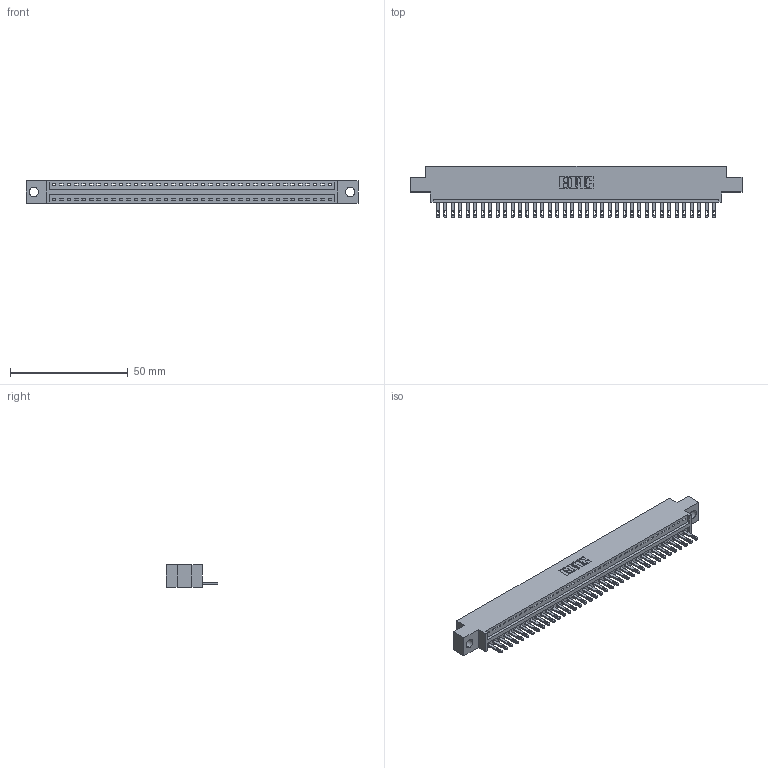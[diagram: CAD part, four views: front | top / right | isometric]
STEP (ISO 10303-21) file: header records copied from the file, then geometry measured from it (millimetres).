
FILE_DESCRIPTION (( 'STEP AP203' ), '1' );
FILE_NAME ('346-038-500-604.STEP', '2022-05-07T04:03:20', ( '' ), ( '' ), 'SwSTEP 2.0', 'SolidWorks 2020', '' );
FILE_SCHEMA (( 'CONFIG_CONTROL_DESIGN' ));
Length unit declared in the file: inch
Products named in the file (3): 346-038-500-604; 346 Part_0.170 Offset - 0.156 Dia-TH; 345-292-001_345-293-100
Assembly tree (39 placements, depth 2):
  346-038-500-604
    346 Part_0.170 Offset - 0.156 Dia-TH
    345-292-001_345-293-100  x38
Bounding box: 141.22 x 21.84 x 9.4 mm (x, y, z)
Volume: 13253.7 mm3; surface area: 16608.3 mm2
Topology: 39 solids, 39 shells, 2192 faces, 6761 edges, 4506 vertices
Faces by surface type: plane 1386, cylinder 806
Entity records: 24603 total; most frequent: CARTESIAN_POINT 4228, ORIENTED_EDGE 4198, DIRECTION 3735, EDGE_CURVE 2099, VECTOR 1811, LINE 1811, VERTEX_POINT 1398, AXIS2_PLACEMENT_3D 962
